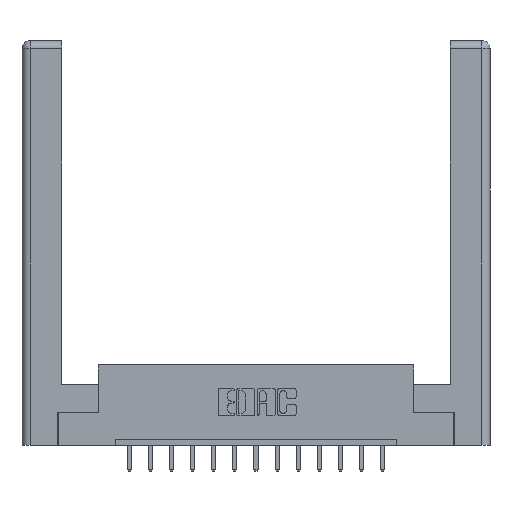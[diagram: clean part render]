
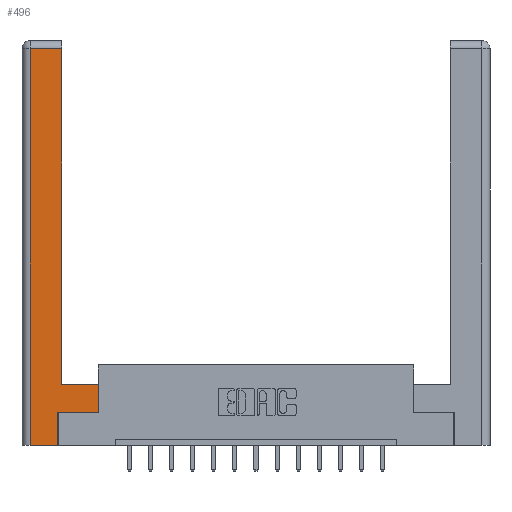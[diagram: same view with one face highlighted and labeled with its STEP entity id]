
A CAD part, top view. The second image highlights one B-rep face of the part: STEP entity #496.
In plain terms, the highlighted planar face has unit normal (0, 0, 1).
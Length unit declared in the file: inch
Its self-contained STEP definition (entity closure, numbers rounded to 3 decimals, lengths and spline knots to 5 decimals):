
#32 = AXIS2_PLACEMENT_3D ( 'NONE', #10518, #15525, #4252 ) ;
#496 = ADVANCED_FACE ( 'NONE', ( #8149 ), #11858, .F. ) ;
#609 = DIRECTION ( 'NONE',  ( 0., -1., 0. ) ) ;
#773 = EDGE_CURVE ( 'NONE', #10136, #3097, #9324, .T. ) ;
#918 = CARTESIAN_POINT ( 'NONE',  ( 0.0615, 2.94, 0. ) ) ;
#948 = DIRECTION ( 'NONE',  ( 0., 1., 0. ) ) ;
#1120 = CARTESIAN_POINT ( 'NONE',  ( 0.565, 0.245, 0. ) ) ;
#1173 = DIRECTION ( 'NONE',  ( 1., 0., 0. ) ) ;
#1411 = ORIENTED_EDGE ( 'NONE', *, *, #10865, .T. ) ;
#2103 = CARTESIAN_POINT ( 'NONE',  ( 0.0615, 0., 0. ) ) ;
#2127 = VERTEX_POINT ( 'NONE', #918 ) ;
#2506 = ORIENTED_EDGE ( 'NONE', *, *, #4572, .T. ) ;
#2580 = DIRECTION ( 'NONE',  ( 1., 0., 0. ) ) ;
#3097 = VERTEX_POINT ( 'NONE', #11452 ) ;
#3268 = EDGE_CURVE ( 'NONE', #9611, #2127, #12180, .T. ) ;
#3652 = CARTESIAN_POINT ( 'NONE',  ( 0.295, 0.45, 0. ) ) ;
#4075 = VECTOR ( 'NONE', #948, 39.37008 ) ;
#4252 = DIRECTION ( 'NONE',  ( -1., 0., 0. ) ) ;
#4470 = ORIENTED_EDGE ( 'NONE', *, *, #9059, .T. ) ;
#4572 = EDGE_CURVE ( 'NONE', #5404, #9611, #15938, .T. ) ;
#4665 = VERTEX_POINT ( 'NONE', #10024 ) ;
#5009 = CARTESIAN_POINT ( 'NONE',  ( 0.0615, 0., 0. ) ) ;
#5335 = ORIENTED_EDGE ( 'NONE', *, *, #14191, .T. ) ;
#5404 = VERTEX_POINT ( 'NONE', #9379 ) ;
#5500 = DIRECTION ( 'NONE',  ( 0., 1., 0. ) ) ;
#5937 = LINE ( 'NONE', #2103, #12780 ) ;
#5996 = EDGE_CURVE ( 'NONE', #2127, #7186, #5937, .T. ) ;
#7186 = VERTEX_POINT ( 'NONE', #5009 ) ;
#7216 = CARTESIAN_POINT ( 'NONE',  ( 0.295, 3., 0. ) ) ;
#7238 = VECTOR ( 'NONE', #5500, 39.37008 ) ;
#7410 = LINE ( 'NONE', #9029, #14850 ) ;
#7966 = EDGE_CURVE ( 'NONE', #12189, #5404, #14505, .T. ) ;
#8008 = CARTESIAN_POINT ( 'NONE',  ( 0.265, 0.245, 0. ) ) ;
#8114 = CARTESIAN_POINT ( 'NONE',  ( 0.295, 2.94, 0. ) ) ;
#8149 = FACE_OUTER_BOUND ( 'NONE', #11450, .T. ) ;
#8660 = CARTESIAN_POINT ( 'NONE',  ( 0.265, 0.245, 0. ) ) ;
#8973 = ORIENTED_EDGE ( 'NONE', *, *, #773, .T. ) ;
#9029 = CARTESIAN_POINT ( 'NONE',  ( 0.265, 0., 0. ) ) ;
#9059 = EDGE_CURVE ( 'NONE', #7186, #4665, #7410, .T. ) ;
#9324 = LINE ( 'NONE', #1120, #13774 ) ;
#9379 = CARTESIAN_POINT ( 'NONE',  ( 0.295, 0.45, 0. ) ) ;
#9390 = ORIENTED_EDGE ( 'NONE', *, *, #3268, .T. ) ;
#9611 = VERTEX_POINT ( 'NONE', #8114 ) ;
#9707 = CARTESIAN_POINT ( 'NONE',  ( 0.565, 0.45, 0. ) ) ;
#9729 = VECTOR ( 'NONE', #12410, 39.37008 ) ;
#10024 = CARTESIAN_POINT ( 'NONE',  ( 0.265, 0., 0. ) ) ;
#10136 = VERTEX_POINT ( 'NONE', #8008 ) ;
#10518 = CARTESIAN_POINT ( 'NONE',  ( 0., 0., 0. ) ) ;
#10865 = EDGE_CURVE ( 'NONE', #4665, #10136, #13821, .T. ) ;
#10995 = ORIENTED_EDGE ( 'NONE', *, *, #7966, .T. ) ;
#11450 = EDGE_LOOP ( 'NONE', ( #2506, #9390, #12824, #4470, #1411, #8973, #5335, #10995 ) ) ;
#11452 = CARTESIAN_POINT ( 'NONE',  ( 0.565, 0.245, 0. ) ) ;
#11858 = PLANE ( 'NONE',  #32 ) ;
#12180 = LINE ( 'NONE', #14448, #14710 ) ;
#12189 = VERTEX_POINT ( 'NONE', #9707 ) ;
#12410 = DIRECTION ( 'NONE',  ( 0., 1., 0. ) ) ;
#12729 = LINE ( 'NONE', #15582, #7238 ) ;
#12780 = VECTOR ( 'NONE', #609, 39.37008 ) ;
#12824 = ORIENTED_EDGE ( 'NONE', *, *, #5996, .T. ) ;
#12940 = VECTOR ( 'NONE', #14872, 39.37008 ) ;
#13774 = VECTOR ( 'NONE', #1173, 39.37008 ) ;
#13821 = LINE ( 'NONE', #8660, #9729 ) ;
#14191 = EDGE_CURVE ( 'NONE', #3097, #12189, #12729, .T. ) ;
#14448 = CARTESIAN_POINT ( 'NONE',  ( 0.0615, 2.94, 0. ) ) ;
#14505 = LINE ( 'NONE', #3652, #12940 ) ;
#14710 = VECTOR ( 'NONE', #15739, 39.37008 ) ;
#14850 = VECTOR ( 'NONE', #2580, 39.37008 ) ;
#14872 = DIRECTION ( 'NONE',  ( -1., 0., 0. ) ) ;
#15525 = DIRECTION ( 'NONE',  ( 0., 0., -1. ) ) ;
#15582 = CARTESIAN_POINT ( 'NONE',  ( 0.565, 0.45, 0. ) ) ;
#15739 = DIRECTION ( 'NONE',  ( -1., 0., 0. ) ) ;
#15938 = LINE ( 'NONE', #7216, #4075 ) ;
